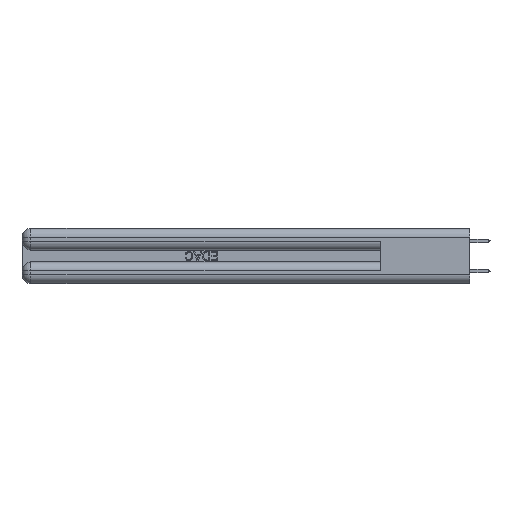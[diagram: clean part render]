
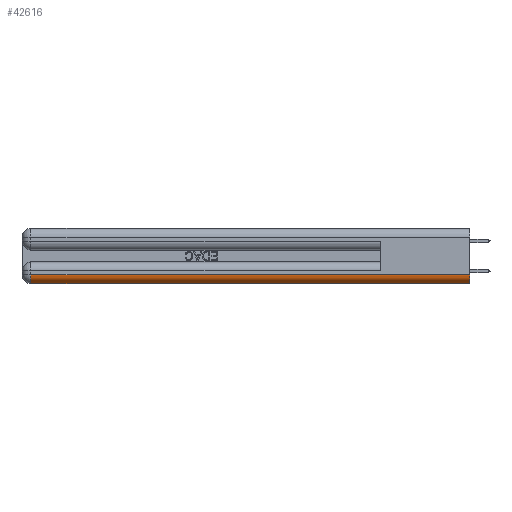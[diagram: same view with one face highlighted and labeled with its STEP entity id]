
A CAD part, left-side view. The second image highlights one B-rep face of the part: STEP entity #42616.
In plain terms, the highlighted cylindrical face has radius 1.524 mm (diameter 3.048 mm), a partial arc.
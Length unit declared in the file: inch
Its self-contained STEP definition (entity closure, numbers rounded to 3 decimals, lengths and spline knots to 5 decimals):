
#569 = CIRCLE ( 'NONE', #10526, 0.06 ) ;
#2280 = DIRECTION ( 'NONE',  ( 0., -1., 0. ) ) ;
#3754 = DIRECTION ( 'NONE',  ( 0., -1., 0. ) ) ;
#5260 = ORIENTED_EDGE ( 'NONE', *, *, #16149, .F. ) ;
#6109 = CYLINDRICAL_SURFACE ( 'NONE', #43286, 0.06 ) ;
#8255 = ORIENTED_EDGE ( 'NONE', *, *, #44332, .F. ) ;
#9179 = LINE ( 'NONE', #18954, #18121 ) ;
#10526 = AXIS2_PLACEMENT_3D ( 'NONE', #44760, #22047, #48536 ) ;
#16149 = EDGE_CURVE ( 'NONE', #43949, #23221, #47278, .T. ) ;
#16827 = CARTESIAN_POINT ( 'NONE',  ( 0.06, 2.94, 0. ) ) ;
#16912 = VERTEX_POINT ( 'NONE', #44127 ) ;
#18121 = VECTOR ( 'NONE', #3754, 39.37008 ) ;
#18954 = CARTESIAN_POINT ( 'NONE',  ( 0., 0., 0.06 ) ) ;
#20166 = ORIENTED_EDGE ( 'NONE', *, *, #37098, .F. ) ;
#20309 = EDGE_CURVE ( 'NONE', #16912, #25629, #9179, .T. ) ;
#22012 = CARTESIAN_POINT ( 'NONE',  ( 0.06, 0., 0.06 ) ) ;
#22047 = DIRECTION ( 'NONE',  ( 0., 1., 0. ) ) ;
#22829 = EDGE_LOOP ( 'NONE', ( #20166, #23755, #8255, #5260 ) ) ;
#23221 = VERTEX_POINT ( 'NONE', #16827 ) ;
#23755 = ORIENTED_EDGE ( 'NONE', *, *, #20309, .F. ) ;
#24309 = CARTESIAN_POINT ( 'NONE',  ( 0.06, 3., 0. ) ) ;
#25145 = CARTESIAN_POINT ( 'NONE',  ( 0.06, 0., 0.06 ) ) ;
#25629 = VERTEX_POINT ( 'NONE', #26046 ) ;
#26046 = CARTESIAN_POINT ( 'NONE',  ( 0., 0., 0.06 ) ) ;
#28189 = DIRECTION ( 'NONE',  ( 0., 1., 0. ) ) ;
#29008 = DIRECTION ( 'NONE',  ( 0., 0., 1. ) ) ;
#30036 = FACE_OUTER_BOUND ( 'NONE', #22829, .T. ) ;
#35560 = CIRCLE ( 'NONE', #39495, 0.06 ) ;
#37098 = EDGE_CURVE ( 'NONE', #25629, #43949, #35560, .T. ) ;
#37134 = DIRECTION ( 'NONE',  ( 0., 1., 0. ) ) ;
#37832 = CARTESIAN_POINT ( 'NONE',  ( 0.06, 0., 0. ) ) ;
#39495 = AXIS2_PLACEMENT_3D ( 'NONE', #25145, #2280, #29008 ) ;
#42616 = ADVANCED_FACE ( 'NONE', ( #30036 ), #6109, .T. ) ;
#43286 = AXIS2_PLACEMENT_3D ( 'NONE', #22012, #37134, #48509 ) ;
#43949 = VERTEX_POINT ( 'NONE', #37832 ) ;
#44127 = CARTESIAN_POINT ( 'NONE',  ( 0., 2.94, 0.06 ) ) ;
#44332 = EDGE_CURVE ( 'NONE', #23221, #16912, #569, .T. ) ;
#44760 = CARTESIAN_POINT ( 'NONE',  ( 0.06, 2.94, 0.06 ) ) ;
#47278 = LINE ( 'NONE', #24309, #48461 ) ;
#48461 = VECTOR ( 'NONE', #28189, 39.37008 ) ;
#48509 = DIRECTION ( 'NONE',  ( 0., 0., 1. ) ) ;
#48536 = DIRECTION ( 'NONE',  ( 0., 0., 1. ) ) ;
